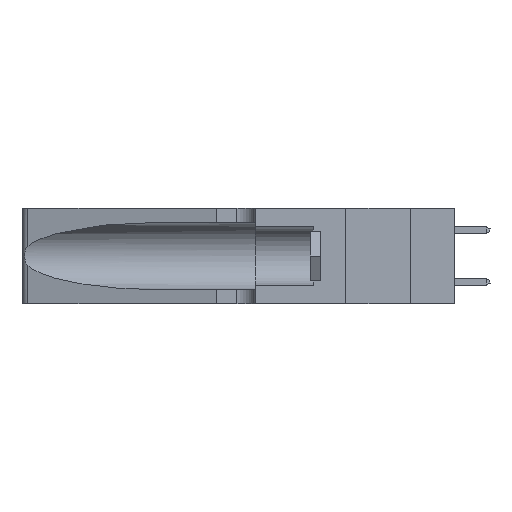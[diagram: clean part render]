
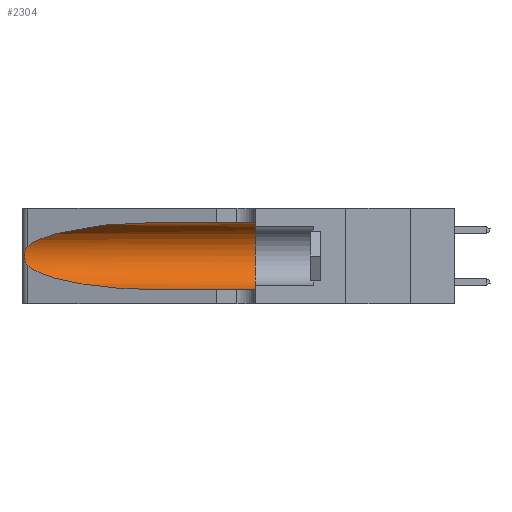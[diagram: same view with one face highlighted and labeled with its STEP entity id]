
A CAD part, left-side view. The second image highlights one B-rep face of the part: STEP entity #2304.
In plain terms, the highlighted cylindrical face has radius 3.308 mm (diameter 6.617 mm), a partial arc.
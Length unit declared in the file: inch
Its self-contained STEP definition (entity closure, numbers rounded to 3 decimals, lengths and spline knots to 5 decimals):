
#681 = CARTESIAN_POINT ( 'NONE',  ( 0.1305, 0.72297, 0.05475 ) ) ;
#816 = ORIENTED_EDGE ( 'NONE', *, *, #12915, .T. ) ;
#1105 = DIRECTION ( 'NONE',  ( 0., 1., 0. ) ) ;
#1185 = AXIS2_PLACEMENT_3D ( 'NONE', #10672, #1105, #9287 ) ;
#1265 = CARTESIAN_POINT ( 'NONE',  ( 0.25487, 1.22718, 0.14631 ) ) ;
#1720 = EDGE_CURVE ( 'NONE', #14225, #11281, #13319, .T. ) ;
#1917 = CARTESIAN_POINT ( 'NONE',  ( 0.25639, 1.23186, 0.15144 ) ) ;
#2287 = VERTEX_POINT ( 'NONE', #7714 ) ;
#2304 = ADVANCED_FACE ( 'NONE', ( #19609 ), #7919, .F. ) ;
#3192 = CARTESIAN_POINT ( 'NONE',  ( 0.1305, 0.72297, 0.05475 ) ) ;
#3417 = CARTESIAN_POINT ( 'NONE',  ( 0.25639, 1.23184, 0.21858 ) ) ;
#3679 = CARTESIAN_POINT ( 'NONE',  ( 0.25856, 1.23593, 0.16098 ) ) ;
#3747 = CARTESIAN_POINT ( 'NONE',  ( 0.25789, 1.23486, 0.15765 ) ) ;
#4135 = CARTESIAN_POINT ( 'NONE',  ( 0.1305, 1.61858, 0.31525 ) ) ;
#4696 = AXIS2_PLACEMENT_3D ( 'NONE', #19086, #19233, #20700 ) ;
#5026 = CARTESIAN_POINT ( 'NONE',  ( 0.25487, 1.22718, 0.14631 ) ) ;
#5725 = VECTOR ( 'NONE', #10594, 39.37008 ) ;
#5774 = LINE ( 'NONE', #5793, #14735 ) ;
#5793 = CARTESIAN_POINT ( 'NONE',  ( 0.1305, 1.61858, 0.05475 ) ) ;
#7359 = CARTESIAN_POINT ( 'NONE',  ( 0.25487, 1.22718, 0.22369 ) ) ;
#7491 = VERTEX_POINT ( 'NONE', #681 ) ;
#7554 = CARTESIAN_POINT ( 'NONE',  ( 0.1305, 0.35, 0.31525 ) ) ;
#7714 = CARTESIAN_POINT ( 'NONE',  ( 0.25487, 1.22718, 0.22369 ) ) ;
#7752 = DIRECTION ( 'NONE',  ( 0., -1., 0. ) ) ;
#7919 = CYLINDRICAL_SURFACE ( 'NONE', #4696, 0.13025 ) ;
#8103 = VERTEX_POINT ( 'NONE', #17534 ) ;
#8924 = ORIENTED_EDGE ( 'NONE', *, *, #1720, .F. ) ;
#9007 = B_SPLINE_CURVE_WITH_KNOTS ( 'NONE', 3,
 ( #7359, #13801, #3417, #14759, #16190, #13410, #19839, #16790, #9983, #3679, #3747, #1917, #13277, #15030 ),
 .UNSPECIFIED., .F., .F.,
 ( 4, 2, 2, 2, 2, 2, 4 ),
 ( 0., 0.00027, 0.00053, 0.00107, 0.0016, 0.00187, 0.00214 ),
 .UNSPECIFIED. ) ;
#9287 = DIRECTION ( 'NONE',  ( 0., 0., 1. ) ) ;
#9950 =( BOUNDED_CURVE ( )  B_SPLINE_CURVE ( 3, ( #16658, #19759, #18130, #18200 ),
 .UNSPECIFIED., .F., .F. ) 
 B_SPLINE_CURVE_WITH_KNOTS ( ( 4, 4 ),
 ( 1.5708, 2.84003 ),
 .UNSPECIFIED. ) 
 CURVE ( )  GEOMETRIC_REPRESENTATION_ITEM ( )  RATIONAL_B_SPLINE_CURVE ( ( 1., 0.87, 0.87, 1. ) ) 
 REPRESENTATION_ITEM ( '' )  );
#9983 = CARTESIAN_POINT ( 'NONE',  ( 0.26017, 1.23833, 0.17102 ) ) ;
#10594 = DIRECTION ( 'NONE',  ( 0., -1., 0. ) ) ;
#10672 = CARTESIAN_POINT ( 'NONE',  ( 0.1305, 0.35, 0.185 ) ) ;
#10917 = EDGE_CURVE ( 'NONE', #8103, #14225, #16696, .T. ) ;
#11055 = CARTESIAN_POINT ( 'NONE',  ( 0.18966, 0.96281, 0.05475 ) ) ;
#11172 = ORIENTED_EDGE ( 'NONE', *, *, #13056, .T. ) ;
#11281 = VERTEX_POINT ( 'NONE', #13419 ) ;
#11926 =( BOUNDED_CURVE ( )  B_SPLINE_CURVE ( 3, ( #1265, #12910, #11055, #3192 ),
 .UNSPECIFIED., .F., .F. ) 
 B_SPLINE_CURVE_WITH_KNOTS ( ( 4, 4 ),
 ( 3.44316, 4.71239 ),
 .UNSPECIFIED. ) 
 CURVE ( )  GEOMETRIC_REPRESENTATION_ITEM ( )  RATIONAL_B_SPLINE_CURVE ( ( 1., 0.87, 0.87, 1. ) ) 
 REPRESENTATION_ITEM ( '' )  );
#12060 = VERTEX_POINT ( 'NONE', #5026 ) ;
#12811 = ORIENTED_EDGE ( 'NONE', *, *, #10917, .F. ) ;
#12910 = CARTESIAN_POINT ( 'NONE',  ( 0.2373, 1.15595, 0.08982 ) ) ;
#12915 = EDGE_CURVE ( 'NONE', #8103, #2287, #9950, .T. ) ;
#13056 = EDGE_CURVE ( 'NONE', #12060, #7491, #11926, .T. ) ;
#13277 = CARTESIAN_POINT ( 'NONE',  ( 0.25555, 1.22993, 0.14849 ) ) ;
#13319 = CIRCLE ( 'NONE', #1185, 0.13025 ) ;
#13410 = CARTESIAN_POINT ( 'NONE',  ( 0.26018, 1.23835, 0.19895 ) ) ;
#13419 = CARTESIAN_POINT ( 'NONE',  ( 0.1305, 0.35, 0.05475 ) ) ;
#13801 = CARTESIAN_POINT ( 'NONE',  ( 0.25555, 1.22994, 0.2215 ) ) ;
#14225 = VERTEX_POINT ( 'NONE', #7554 ) ;
#14615 = EDGE_CURVE ( 'NONE', #2287, #12060, #9007, .T. ) ;
#14735 = VECTOR ( 'NONE', #7752, 39.37008 ) ;
#14759 = CARTESIAN_POINT ( 'NONE',  ( 0.25787, 1.23484, 0.2124 ) ) ;
#15030 = CARTESIAN_POINT ( 'NONE',  ( 0.25487, 1.22718, 0.14631 ) ) ;
#15635 = EDGE_LOOP ( 'NONE', ( #816, #18862, #11172, #20846, #8924, #12811 ) ) ;
#16190 = CARTESIAN_POINT ( 'NONE',  ( 0.25854, 1.2359, 0.20912 ) ) ;
#16658 = CARTESIAN_POINT ( 'NONE',  ( 0.1305, 0.72297, 0.31525 ) ) ;
#16696 = LINE ( 'NONE', #4135, #5725 ) ;
#16790 = CARTESIAN_POINT ( 'NONE',  ( 0.26075, 1.23896, 0.178 ) ) ;
#17534 = CARTESIAN_POINT ( 'NONE',  ( 0.1305, 0.72297, 0.31525 ) ) ;
#18080 = EDGE_CURVE ( 'NONE', #7491, #11281, #5774, .T. ) ;
#18130 = CARTESIAN_POINT ( 'NONE',  ( 0.2373, 1.15595, 0.28018 ) ) ;
#18200 = CARTESIAN_POINT ( 'NONE',  ( 0.25487, 1.22718, 0.22369 ) ) ;
#18862 = ORIENTED_EDGE ( 'NONE', *, *, #14615, .T. ) ;
#19086 = CARTESIAN_POINT ( 'NONE',  ( 0.1305, 1.61858, 0.185 ) ) ;
#19233 = DIRECTION ( 'NONE',  ( 0., -1., 0. ) ) ;
#19609 = FACE_OUTER_BOUND ( 'NONE', #15635, .T. ) ;
#19759 = CARTESIAN_POINT ( 'NONE',  ( 0.18966, 0.96281, 0.31525 ) ) ;
#19839 = CARTESIAN_POINT ( 'NONE',  ( 0.26075, 1.23896, 0.19203 ) ) ;
#20700 = DIRECTION ( 'NONE',  ( 0., 0., -1. ) ) ;
#20846 = ORIENTED_EDGE ( 'NONE', *, *, #18080, .T. ) ;
